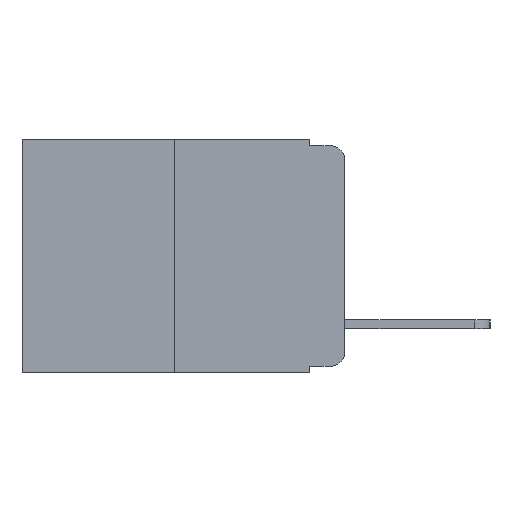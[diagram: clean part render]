
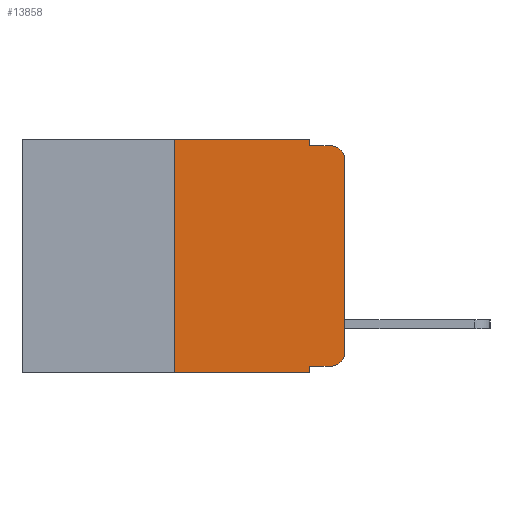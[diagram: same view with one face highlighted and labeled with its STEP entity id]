
A CAD part, left-side view. The second image highlights one B-rep face of the part: STEP entity #13858.
In plain terms, the highlighted planar face has unit normal (-1, 0, 0).
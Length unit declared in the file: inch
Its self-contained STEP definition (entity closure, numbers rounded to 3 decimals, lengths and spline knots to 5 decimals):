
#319 = VECTOR ( 'NONE', #9718, 39.37008 ) ;
#565 = VERTEX_POINT ( 'NONE', #16682 ) ;
#591 = AXIS2_PLACEMENT_3D ( 'NONE', #13249, #16453, #16403 ) ;
#689 = DIRECTION ( 'NONE',  ( -1., 0., 0. ) ) ;
#1806 = VERTEX_POINT ( 'NONE', #4047 ) ;
#2147 = LINE ( 'NONE', #16803, #13295 ) ;
#2872 = ORIENTED_EDGE ( 'NONE', *, *, #13462, .T. ) ;
#3269 = DIRECTION ( 'NONE',  ( 0., 0., 1. ) ) ;
#3355 = DIRECTION ( 'NONE',  ( 0., 0., -1. ) ) ;
#3386 = ORIENTED_EDGE ( 'NONE', *, *, #4045, .T. ) ;
#3590 = LINE ( 'NONE', #12891, #6535 ) ;
#3778 = EDGE_CURVE ( 'NONE', #13764, #10708, #14944, .T. ) ;
#3860 = EDGE_CURVE ( 'NONE', #1806, #13764, #2147, .T. ) ;
#3863 = EDGE_CURVE ( 'NONE', #565, #6454, #16851, .T. ) ;
#3993 = EDGE_CURVE ( 'NONE', #6777, #9482, #14726, .T. ) ;
#4045 = EDGE_CURVE ( 'NONE', #6777, #12447, #17045, .T. ) ;
#4047 = CARTESIAN_POINT ( 'NONE',  ( 0., 0.051, 0. ) ) ;
#4163 = EDGE_LOOP ( 'NONE', ( #9157, #9597, #13045, #6324, #9983, #13468, #2872, #6813, #3386, #7250 ) ) ;
#4241 = EDGE_CURVE ( 'NONE', #12447, #8163, #8331, .T. ) ;
#4476 = EDGE_CURVE ( 'NONE', #6454, #1806, #6108, .T. ) ;
#5102 = CIRCLE ( 'NONE', #13515, 0.02 ) ;
#5394 = DIRECTION ( 'NONE',  ( 0., -1., 0. ) ) ;
#5633 = CARTESIAN_POINT ( 'NONE',  ( 0., 0.473, 0. ) ) ;
#5682 = VECTOR ( 'NONE', #7752, 39.37008 ) ;
#6108 = LINE ( 'NONE', #5633, #5682 ) ;
#6324 = ORIENTED_EDGE ( 'NONE', *, *, #3860, .F. ) ;
#6377 = DIRECTION ( 'NONE',  ( 0., 0., -1. ) ) ;
#6379 = EDGE_CURVE ( 'NONE', #8163, #8471, #3590, .T. ) ;
#6454 = VERTEX_POINT ( 'NONE', #11717 ) ;
#6535 = VECTOR ( 'NONE', #3269, 39.37008 ) ;
#6777 = VERTEX_POINT ( 'NONE', #7723 ) ;
#6813 = ORIENTED_EDGE ( 'NONE', *, *, #3993, .F. ) ;
#7250 = ORIENTED_EDGE ( 'NONE', *, *, #4241, .T. ) ;
#7723 = CARTESIAN_POINT ( 'NONE',  ( 0., 0.051, -0.333 ) ) ;
#7752 = DIRECTION ( 'NONE',  ( 0., -1., 0. ) ) ;
#8090 = EDGE_CURVE ( 'NONE', #8471, #10708, #5102, .T. ) ;
#8163 = VERTEX_POINT ( 'NONE', #17584 ) ;
#8331 = CIRCLE ( 'NONE', #591, 0.02 ) ;
#8471 = VERTEX_POINT ( 'NONE', #16636 ) ;
#9157 = ORIENTED_EDGE ( 'NONE', *, *, #6379, .T. ) ;
#9419 = VECTOR ( 'NONE', #13020, 39.37008 ) ;
#9482 = VERTEX_POINT ( 'NONE', #15704 ) ;
#9563 = CARTESIAN_POINT ( 'NONE',  ( 0., 0.02, -0.03 ) ) ;
#9597 = ORIENTED_EDGE ( 'NONE', *, *, #8090, .T. ) ;
#9681 = FACE_OUTER_BOUND ( 'NONE', #4163, .T. ) ;
#9718 = DIRECTION ( 'NONE',  ( 0., -1., 0. ) ) ;
#9983 = ORIENTED_EDGE ( 'NONE', *, *, #4476, .F. ) ;
#10347 = PLANE ( 'NONE',  #12777 ) ;
#10708 = VERTEX_POINT ( 'NONE', #15629 ) ;
#10899 = DIRECTION ( 'NONE',  ( 0., 0., -1. ) ) ;
#11245 = DIRECTION ( 'NONE',  ( 0., -1., 0. ) ) ;
#11335 = CARTESIAN_POINT ( 'NONE',  ( 0., 0.051, -0.333 ) ) ;
#11552 = CARTESIAN_POINT ( 'NONE',  ( 0., 0.02, -0.333 ) ) ;
#11683 = DIRECTION ( 'NONE',  ( 1., 0., 0. ) ) ;
#11717 = CARTESIAN_POINT ( 'NONE',  ( 0., 0.25, 0. ) ) ;
#12447 = VERTEX_POINT ( 'NONE', #11552 ) ;
#12510 = CARTESIAN_POINT ( 'NONE',  ( 0., 0.051, -0.01 ) ) ;
#12743 = VECTOR ( 'NONE', #5394, 39.37008 ) ;
#12748 = CARTESIAN_POINT ( 'NONE',  ( 0., 0.051, -0.01 ) ) ;
#12777 = AXIS2_PLACEMENT_3D ( 'NONE', #15585, #11683, #3355 ) ;
#12891 = CARTESIAN_POINT ( 'NONE',  ( 0., 0., 0. ) ) ;
#13020 = DIRECTION ( 'NONE',  ( 0., 0., 1. ) ) ;
#13045 = ORIENTED_EDGE ( 'NONE', *, *, #3778, .F. ) ;
#13249 = CARTESIAN_POINT ( 'NONE',  ( 0., 0.02, -0.313 ) ) ;
#13295 = VECTOR ( 'NONE', #6377, 39.37008 ) ;
#13462 = EDGE_CURVE ( 'NONE', #565, #9482, #16273, .T. ) ;
#13468 = ORIENTED_EDGE ( 'NONE', *, *, #3863, .F. ) ;
#13489 = VECTOR ( 'NONE', #11245, 39.37008 ) ;
#13515 = AXIS2_PLACEMENT_3D ( 'NONE', #9563, #689, #10899 ) ;
#13764 = VERTEX_POINT ( 'NONE', #12748 ) ;
#13858 = ADVANCED_FACE ( 'NONE', ( #9681 ), #10347, .F. ) ;
#14319 = VECTOR ( 'NONE', #14582, 39.37008 ) ;
#14582 = DIRECTION ( 'NONE',  ( 0., 0., -1. ) ) ;
#14726 = LINE ( 'NONE', #14955, #14319 ) ;
#14779 = CARTESIAN_POINT ( 'NONE',  ( 0., 0.473, -0.343 ) ) ;
#14944 = LINE ( 'NONE', #12510, #319 ) ;
#14955 = CARTESIAN_POINT ( 'NONE',  ( 0., 0.051, 0. ) ) ;
#15585 = CARTESIAN_POINT ( 'NONE',  ( 0., 0.473, 0. ) ) ;
#15629 = CARTESIAN_POINT ( 'NONE',  ( 0., 0.02, -0.01 ) ) ;
#15704 = CARTESIAN_POINT ( 'NONE',  ( 0., 0.051, -0.343 ) ) ;
#16273 = LINE ( 'NONE', #14779, #12743 ) ;
#16403 = DIRECTION ( 'NONE',  ( 0., 0., -1. ) ) ;
#16453 = DIRECTION ( 'NONE',  ( -1., 0., 0. ) ) ;
#16636 = CARTESIAN_POINT ( 'NONE',  ( 0., 0., -0.03 ) ) ;
#16682 = CARTESIAN_POINT ( 'NONE',  ( 0., 0.25, -0.343 ) ) ;
#16803 = CARTESIAN_POINT ( 'NONE',  ( 0., 0.051, 0. ) ) ;
#16851 = LINE ( 'NONE', #18106, #9419 ) ;
#17045 = LINE ( 'NONE', #11335, #13489 ) ;
#17584 = CARTESIAN_POINT ( 'NONE',  ( 0., 0., -0.313 ) ) ;
#18106 = CARTESIAN_POINT ( 'NONE',  ( 0., 0.25, 0. ) ) ;
